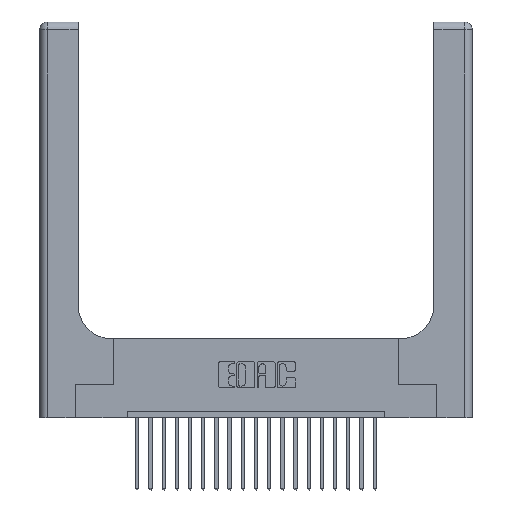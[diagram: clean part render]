
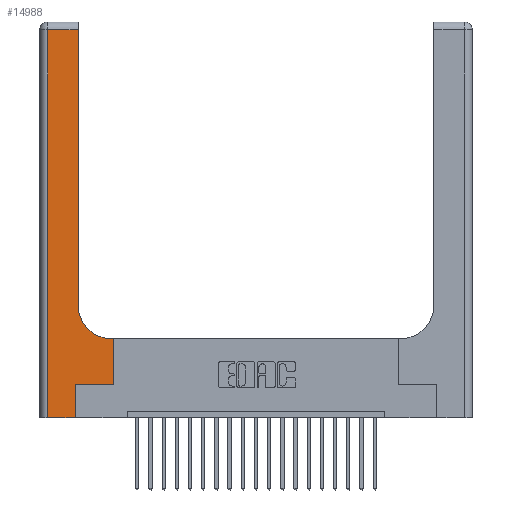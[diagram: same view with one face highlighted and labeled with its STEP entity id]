
A CAD part, top view. The second image highlights one B-rep face of the part: STEP entity #14988.
In plain terms, the highlighted planar face has unit normal (0, 0, 1).
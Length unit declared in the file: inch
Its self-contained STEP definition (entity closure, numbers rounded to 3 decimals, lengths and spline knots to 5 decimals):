
#11 = VERTEX_POINT ( 'NONE', #1510 ) ;
#99 = CARTESIAN_POINT ( 'NONE',  ( 0.269, 0.25, 0.37 ) ) ;
#347 = CARTESIAN_POINT ( 'NONE',  ( 0.06, 2.94, 0.37 ) ) ;
#423 = DIRECTION ( 'NONE',  ( 0., 0., -1. ) ) ;
#757 = VECTOR ( 'NONE', #1476, 39.37008 ) ;
#959 = CARTESIAN_POINT ( 'NONE',  ( 0.269, 0., 0.37 ) ) ;
#1092 = LINE ( 'NONE', #17520, #18574 ) ;
#1123 = CARTESIAN_POINT ( 'NONE',  ( 0.5585, 0.6, 0.37 ) ) ;
#1240 = ORIENTED_EDGE ( 'NONE', *, *, #12994, .T. ) ;
#1349 = EDGE_CURVE ( 'NONE', #12143, #3382, #20994, .T. ) ;
#1476 = DIRECTION ( 'NONE',  ( 0., -1., 0. ) ) ;
#1488 = CARTESIAN_POINT ( 'NONE',  ( 0.269, 0.25, 0.37 ) ) ;
#1510 = CARTESIAN_POINT ( 'NONE',  ( 0.2915, 0.85, 0.37 ) ) ;
#1614 = EDGE_CURVE ( 'NONE', #11, #12143, #1092, .T. ) ;
#1845 = ORIENTED_EDGE ( 'NONE', *, *, #13261, .T. ) ;
#2189 = PLANE ( 'NONE',  #5432 ) ;
#2536 = VERTEX_POINT ( 'NONE', #1488 ) ;
#2657 = LINE ( 'NONE', #19464, #17411 ) ;
#2879 = EDGE_CURVE ( 'NONE', #10286, #16103, #2657, .T. ) ;
#3153 = VERTEX_POINT ( 'NONE', #9911 ) ;
#3382 = VERTEX_POINT ( 'NONE', #347 ) ;
#3828 = ORIENTED_EDGE ( 'NONE', *, *, #4797, .T. ) ;
#4595 = VECTOR ( 'NONE', #4655, 39.37008 ) ;
#4655 = DIRECTION ( 'NONE',  ( 1., 0., 0. ) ) ;
#4797 = EDGE_CURVE ( 'NONE', #3153, #10286, #12641, .T. ) ;
#5040 = CARTESIAN_POINT ( 'NONE',  ( 0.5415, 0.85, 0.37 ) ) ;
#5294 = EDGE_CURVE ( 'NONE', #15025, #2536, #20518, .T. ) ;
#5432 = AXIS2_PLACEMENT_3D ( 'NONE', #10876, #423, #12631 ) ;
#5957 = ORIENTED_EDGE ( 'NONE', *, *, #2879, .T. ) ;
#6227 = ORIENTED_EDGE ( 'NONE', *, *, #5294, .T. ) ;
#6595 = DIRECTION ( 'NONE',  ( 1., 0., 0. ) ) ;
#7508 = LINE ( 'NONE', #99, #20854 ) ;
#8339 = AXIS2_PLACEMENT_3D ( 'NONE', #5040, #17053, #6595 ) ;
#9155 = ORIENTED_EDGE ( 'NONE', *, *, #1349, .T. ) ;
#9500 = ORIENTED_EDGE ( 'NONE', *, *, #21463, .T. ) ;
#9503 = CARTESIAN_POINT ( 'NONE',  ( 0.5415, 0.6, 0.37 ) ) ;
#9852 = CARTESIAN_POINT ( 'NONE',  ( 0., 0., 0.37 ) ) ;
#9911 = CARTESIAN_POINT ( 'NONE',  ( 0.5585, 0.25, 0.37 ) ) ;
#10286 = VERTEX_POINT ( 'NONE', #1123 ) ;
#10390 = DIRECTION ( 'NONE',  ( 1., 0., 0. ) ) ;
#10876 = CARTESIAN_POINT ( 'NONE',  ( 0., 3., 0.37 ) ) ;
#10981 = VECTOR ( 'NONE', #13876, 39.37008 ) ;
#11291 = CARTESIAN_POINT ( 'NONE',  ( 0.2915, 2.94, 0.37 ) ) ;
#11842 = CARTESIAN_POINT ( 'NONE',  ( 0.06, 0., 0.37 ) ) ;
#11977 = LINE ( 'NONE', #9852, #4595 ) ;
#12143 = VERTEX_POINT ( 'NONE', #11291 ) ;
#12616 = ORIENTED_EDGE ( 'NONE', *, *, #18713, .T. ) ;
#12631 = DIRECTION ( 'NONE',  ( -1., 0., 0. ) ) ;
#12641 = LINE ( 'NONE', #22622, #14274 ) ;
#12769 = LINE ( 'NONE', #22081, #757 ) ;
#12994 = EDGE_CURVE ( 'NONE', #3382, #13289, #12769, .T. ) ;
#13029 = ORIENTED_EDGE ( 'NONE', *, *, #1614, .T. ) ;
#13261 = EDGE_CURVE ( 'NONE', #16103, #11, #19317, .T. ) ;
#13289 = VERTEX_POINT ( 'NONE', #11842 ) ;
#13876 = DIRECTION ( 'NONE',  ( 0., 1., 0. ) ) ;
#14274 = VECTOR ( 'NONE', #15448, 39.37008 ) ;
#14439 = DIRECTION ( 'NONE',  ( -1., 0., 0. ) ) ;
#14988 = ADVANCED_FACE ( 'NONE', ( #19205 ), #2189, .F. ) ;
#15025 = VERTEX_POINT ( 'NONE', #17760 ) ;
#15448 = DIRECTION ( 'NONE',  ( 0., 1., 0. ) ) ;
#15959 = EDGE_LOOP ( 'NONE', ( #13029, #9155, #1240, #12616, #6227, #9500, #3828, #5957, #1845 ) ) ;
#16103 = VERTEX_POINT ( 'NONE', #9503 ) ;
#17053 = DIRECTION ( 'NONE',  ( 0., 0., -1. ) ) ;
#17411 = VECTOR ( 'NONE', #14439, 39.37008 ) ;
#17520 = CARTESIAN_POINT ( 'NONE',  ( 0.2915, 3., 0.37 ) ) ;
#17760 = CARTESIAN_POINT ( 'NONE',  ( 0.269, 0., 0.37 ) ) ;
#18574 = VECTOR ( 'NONE', #18942, 39.37008 ) ;
#18713 = EDGE_CURVE ( 'NONE', #13289, #15025, #11977, .T. ) ;
#18942 = DIRECTION ( 'NONE',  ( 0., 1., 0. ) ) ;
#19205 = FACE_OUTER_BOUND ( 'NONE', #15959, .T. ) ;
#19317 = CIRCLE ( 'NONE', #8339, 0.25 ) ;
#19344 = VECTOR ( 'NONE', #20976, 39.37008 ) ;
#19464 = CARTESIAN_POINT ( 'NONE',  ( 0.2915, 0.6, 0.37 ) ) ;
#20518 = LINE ( 'NONE', #959, #10981 ) ;
#20854 = VECTOR ( 'NONE', #10390, 39.37008 ) ;
#20976 = DIRECTION ( 'NONE',  ( -1., 0., 0. ) ) ;
#20994 = LINE ( 'NONE', #22503, #19344 ) ;
#21463 = EDGE_CURVE ( 'NONE', #2536, #3153, #7508, .T. ) ;
#22081 = CARTESIAN_POINT ( 'NONE',  ( 0.06, 3., 0.37 ) ) ;
#22503 = CARTESIAN_POINT ( 'NONE',  ( 0., 2.94, 0.37 ) ) ;
#22622 = CARTESIAN_POINT ( 'NONE',  ( 0.5585, 0.25, 0.37 ) ) ;
